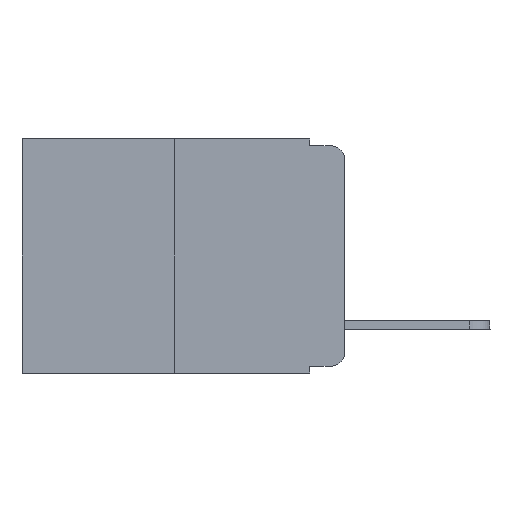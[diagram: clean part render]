
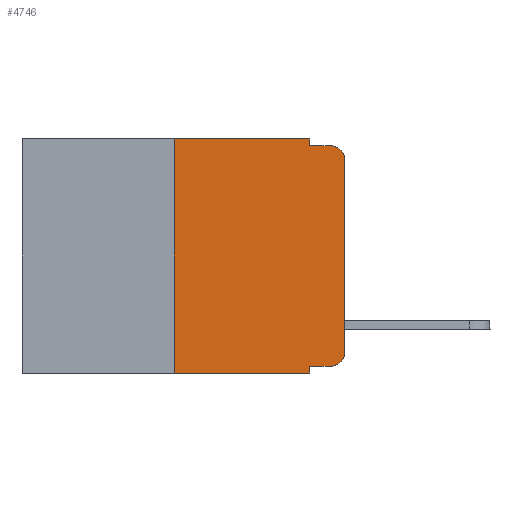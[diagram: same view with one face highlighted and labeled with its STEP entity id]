
A CAD part, left-side view. The second image highlights one B-rep face of the part: STEP entity #4746.
In plain terms, the highlighted planar face has unit normal (-1, 0, 0).
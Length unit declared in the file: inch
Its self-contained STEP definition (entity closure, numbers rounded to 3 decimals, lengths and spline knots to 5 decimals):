
#681 = CARTESIAN_POINT ( 'NONE',  ( 0., 0.25, -0.343 ) ) ;
#736 = CARTESIAN_POINT ( 'NONE',  ( 0., 0., 0. ) ) ;
#811 = LINE ( 'NONE', #10737, #7353 ) ;
#1432 = DIRECTION ( 'NONE',  ( 0., 0., -1. ) ) ;
#1436 = CARTESIAN_POINT ( 'NONE',  ( 0., 0.25, 0. ) ) ;
#1463 = CIRCLE ( 'NONE', #6732, 0.02 ) ;
#1639 = EDGE_CURVE ( 'NONE', #12889, #3578, #14822, .T. ) ;
#2014 = VERTEX_POINT ( 'NONE', #4799 ) ;
#2453 = EDGE_CURVE ( 'NONE', #9601, #3578, #811, .T. ) ;
#2716 = VECTOR ( 'NONE', #5786, 39.37008 ) ;
#2811 = EDGE_LOOP ( 'NONE', ( #7793, #10433, #16198, #12484, #4058, #12455, #12786, #16065, #4981, #13515 ) ) ;
#2870 = CARTESIAN_POINT ( 'NONE',  ( 0., 0.051, 0. ) ) ;
#3028 = DIRECTION ( 'NONE',  ( 0., 0., -1. ) ) ;
#3220 = VECTOR ( 'NONE', #12645, 39.37008 ) ;
#3578 = VERTEX_POINT ( 'NONE', #9137 ) ;
#4030 = CARTESIAN_POINT ( 'NONE',  ( 0., 0.051, -0.333 ) ) ;
#4058 = ORIENTED_EDGE ( 'NONE', *, *, #15861, .F. ) ;
#4746 = ADVANCED_FACE ( 'NONE', ( #14720 ), #8577, .F. ) ;
#4778 = DIRECTION ( 'NONE',  ( 0., 0., -1. ) ) ;
#4799 = CARTESIAN_POINT ( 'NONE',  ( 0., 0.051, -0.01 ) ) ;
#4843 = DIRECTION ( 'NONE',  ( 1., 0., 0. ) ) ;
#4894 = VERTEX_POINT ( 'NONE', #10964 ) ;
#4930 = CARTESIAN_POINT ( 'NONE',  ( 0., 0.02, -0.333 ) ) ;
#4981 = ORIENTED_EDGE ( 'NONE', *, *, #9943, .T. ) ;
#5319 = CIRCLE ( 'NONE', #8748, 0.02 ) ;
#5323 = CARTESIAN_POINT ( 'NONE',  ( 0., 0.051, -0.333 ) ) ;
#5377 = CARTESIAN_POINT ( 'NONE',  ( 0., 0.02, -0.01 ) ) ;
#5786 = DIRECTION ( 'NONE',  ( 0., 0., 1. ) ) ;
#5870 = DIRECTION ( 'NONE',  ( 0., -1., 0. ) ) ;
#6028 = AXIS2_PLACEMENT_3D ( 'NONE', #7334, #4843, #14633 ) ;
#6164 = LINE ( 'NONE', #14956, #12822 ) ;
#6402 = CARTESIAN_POINT ( 'NONE',  ( 0., 0.473, 0. ) ) ;
#6732 = AXIS2_PLACEMENT_3D ( 'NONE', #8085, #14315, #3028 ) ;
#7253 = VERTEX_POINT ( 'NONE', #4930 ) ;
#7334 = CARTESIAN_POINT ( 'NONE',  ( 0., 0.473, 0. ) ) ;
#7353 = VECTOR ( 'NONE', #5870, 39.37008 ) ;
#7418 = LINE ( 'NONE', #736, #2716 ) ;
#7636 = CARTESIAN_POINT ( 'NONE',  ( 0., 0.051, -0.01 ) ) ;
#7793 = ORIENTED_EDGE ( 'NONE', *, *, #12465, .T. ) ;
#8004 = LINE ( 'NONE', #6402, #13861 ) ;
#8085 = CARTESIAN_POINT ( 'NONE',  ( 0., 0.02, -0.03 ) ) ;
#8267 = EDGE_CURVE ( 'NONE', #7253, #8904, #5319, .T. ) ;
#8577 = PLANE ( 'NONE',  #6028 ) ;
#8748 = AXIS2_PLACEMENT_3D ( 'NONE', #11404, #10188, #1432 ) ;
#8801 = VECTOR ( 'NONE', #15378, 39.37008 ) ;
#8815 = DIRECTION ( 'NONE',  ( 0., 0., 1. ) ) ;
#8904 = VERTEX_POINT ( 'NONE', #11265 ) ;
#8956 = LINE ( 'NONE', #2870, #10941 ) ;
#9137 = CARTESIAN_POINT ( 'NONE',  ( 0., 0.051, -0.343 ) ) ;
#9601 = VERTEX_POINT ( 'NONE', #681 ) ;
#9657 = VECTOR ( 'NONE', #4778, 39.37008 ) ;
#9943 = EDGE_CURVE ( 'NONE', #12889, #7253, #15299, .T. ) ;
#10188 = DIRECTION ( 'NONE',  ( -1., 0., 0. ) ) ;
#10208 = EDGE_CURVE ( 'NONE', #2014, #11087, #13877, .T. ) ;
#10421 = DIRECTION ( 'NONE',  ( 0., 0., -1. ) ) ;
#10433 = ORIENTED_EDGE ( 'NONE', *, *, #13347, .T. ) ;
#10580 = DIRECTION ( 'NONE',  ( 0., -1., 0. ) ) ;
#10737 = CARTESIAN_POINT ( 'NONE',  ( 0., 0.473, -0.343 ) ) ;
#10941 = VECTOR ( 'NONE', #10421, 39.37008 ) ;
#10964 = CARTESIAN_POINT ( 'NONE',  ( 0., 0.051, 0. ) ) ;
#11087 = VERTEX_POINT ( 'NONE', #5377 ) ;
#11265 = CARTESIAN_POINT ( 'NONE',  ( 0., 0., -0.313 ) ) ;
#11404 = CARTESIAN_POINT ( 'NONE',  ( 0., 0.02, -0.313 ) ) ;
#11727 = VERTEX_POINT ( 'NONE', #1436 ) ;
#12455 = ORIENTED_EDGE ( 'NONE', *, *, #15408, .F. ) ;
#12465 = EDGE_CURVE ( 'NONE', #8904, #15348, #7418, .T. ) ;
#12484 = ORIENTED_EDGE ( 'NONE', *, *, #13223, .F. ) ;
#12645 = DIRECTION ( 'NONE',  ( 0., -1., 0. ) ) ;
#12786 = ORIENTED_EDGE ( 'NONE', *, *, #2453, .T. ) ;
#12822 = VECTOR ( 'NONE', #8815, 39.37008 ) ;
#12889 = VERTEX_POINT ( 'NONE', #5323 ) ;
#13223 = EDGE_CURVE ( 'NONE', #4894, #2014, #8956, .T. ) ;
#13347 = EDGE_CURVE ( 'NONE', #15348, #11087, #1463, .T. ) ;
#13515 = ORIENTED_EDGE ( 'NONE', *, *, #8267, .T. ) ;
#13861 = VECTOR ( 'NONE', #10580, 39.37008 ) ;
#13877 = LINE ( 'NONE', #7636, #3220 ) ;
#14315 = DIRECTION ( 'NONE',  ( -1., 0., 0. ) ) ;
#14633 = DIRECTION ( 'NONE',  ( 0., 0., -1. ) ) ;
#14720 = FACE_OUTER_BOUND ( 'NONE', #2811, .T. ) ;
#14822 = LINE ( 'NONE', #15958, #9657 ) ;
#14956 = CARTESIAN_POINT ( 'NONE',  ( 0., 0.25, 0. ) ) ;
#15299 = LINE ( 'NONE', #4030, #8801 ) ;
#15348 = VERTEX_POINT ( 'NONE', #16162 ) ;
#15378 = DIRECTION ( 'NONE',  ( 0., -1., 0. ) ) ;
#15408 = EDGE_CURVE ( 'NONE', #9601, #11727, #6164, .T. ) ;
#15861 = EDGE_CURVE ( 'NONE', #11727, #4894, #8004, .T. ) ;
#15958 = CARTESIAN_POINT ( 'NONE',  ( 0., 0.051, 0. ) ) ;
#16065 = ORIENTED_EDGE ( 'NONE', *, *, #1639, .F. ) ;
#16162 = CARTESIAN_POINT ( 'NONE',  ( 0., 0., -0.03 ) ) ;
#16198 = ORIENTED_EDGE ( 'NONE', *, *, #10208, .F. ) ;
